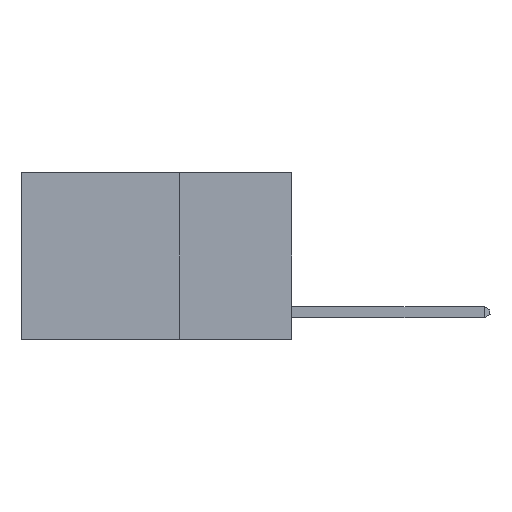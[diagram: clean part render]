
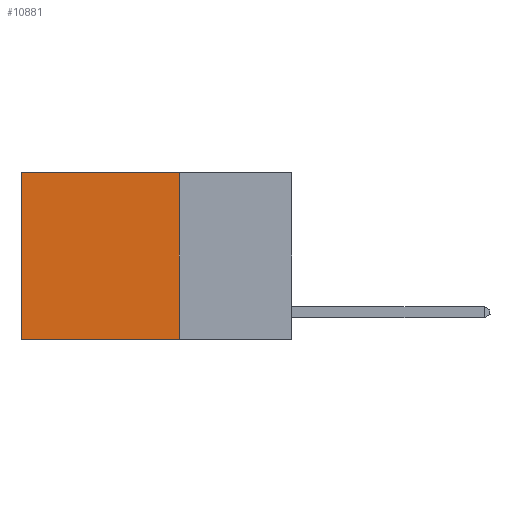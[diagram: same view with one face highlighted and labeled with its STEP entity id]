
A CAD part, left-side view. The second image highlights one B-rep face of the part: STEP entity #10881.
In plain terms, the highlighted planar face has unit normal (-1, 0, 0).
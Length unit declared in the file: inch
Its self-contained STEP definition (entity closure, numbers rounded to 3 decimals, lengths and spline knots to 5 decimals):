
#87 = VERTEX_POINT ( 'NONE', #7663 ) ;
#259 = CARTESIAN_POINT ( 'NONE',  ( 0.2625, 0.25, -0.37 ) ) ;
#1043 = VECTOR ( 'NONE', #4573, 39.37008 ) ;
#1085 = CARTESIAN_POINT ( 'NONE',  ( 0.2625, 0.25, 0. ) ) ;
#1716 = VERTEX_POINT ( 'NONE', #12258 ) ;
#1959 = EDGE_CURVE ( 'NONE', #1716, #6871, #7795, .T. ) ;
#2144 = EDGE_CURVE ( 'NONE', #8159, #6871, #9756, .T. ) ;
#2399 = DIRECTION ( 'NONE',  ( 0., 0., -1. ) ) ;
#3251 = DIRECTION ( 'NONE',  ( 0., 0., -1. ) ) ;
#3423 = EDGE_LOOP ( 'NONE', ( #3823, #11827, #11623, #7044 ) ) ;
#3823 = ORIENTED_EDGE ( 'NONE', *, *, #1959, .T. ) ;
#4270 = LINE ( 'NONE', #8259, #9329 ) ;
#4301 = DIRECTION ( 'NONE',  ( 1., 0., 0. ) ) ;
#4573 = DIRECTION ( 'NONE',  ( 0., 1., 0. ) ) ;
#5570 = DIRECTION ( 'NONE',  ( 0., 0., -1. ) ) ;
#6783 = VECTOR ( 'NONE', #5570, 39.37008 ) ;
#6871 = VERTEX_POINT ( 'NONE', #9048 ) ;
#7044 = ORIENTED_EDGE ( 'NONE', *, *, #11097, .T. ) ;
#7122 = EDGE_CURVE ( 'NONE', #87, #8159, #9806, .T. ) ;
#7663 = CARTESIAN_POINT ( 'NONE',  ( 0.2625, 0.25, 0. ) ) ;
#7795 = LINE ( 'NONE', #12032, #11796 ) ;
#8048 = CARTESIAN_POINT ( 'NONE',  ( 0.2625, 0.25, -0.37 ) ) ;
#8159 = VERTEX_POINT ( 'NONE', #8048 ) ;
#8259 = CARTESIAN_POINT ( 'NONE',  ( 0.2625, 0.25, 0. ) ) ;
#8540 = DIRECTION ( 'NONE',  ( 0., 1., 0. ) ) ;
#8636 = AXIS2_PLACEMENT_3D ( 'NONE', #9561, #4301, #3251 ) ;
#9048 = CARTESIAN_POINT ( 'NONE',  ( 0.2625, 0.6, -0.37 ) ) ;
#9329 = VECTOR ( 'NONE', #8540, 39.37008 ) ;
#9561 = CARTESIAN_POINT ( 'NONE',  ( 0.2625, 0.25, 0. ) ) ;
#9756 = LINE ( 'NONE', #259, #1043 ) ;
#9806 = LINE ( 'NONE', #1085, #6783 ) ;
#10881 = ADVANCED_FACE ( 'NONE', ( #13881 ), #13815, .F. ) ;
#11097 = EDGE_CURVE ( 'NONE', #87, #1716, #4270, .T. ) ;
#11623 = ORIENTED_EDGE ( 'NONE', *, *, #7122, .F. ) ;
#11796 = VECTOR ( 'NONE', #2399, 39.37008 ) ;
#11827 = ORIENTED_EDGE ( 'NONE', *, *, #2144, .F. ) ;
#12032 = CARTESIAN_POINT ( 'NONE',  ( 0.2625, 0.6, 0. ) ) ;
#12258 = CARTESIAN_POINT ( 'NONE',  ( 0.2625, 0.6, 0. ) ) ;
#13815 = PLANE ( 'NONE',  #8636 ) ;
#13881 = FACE_OUTER_BOUND ( 'NONE', #3423, .T. ) ;
